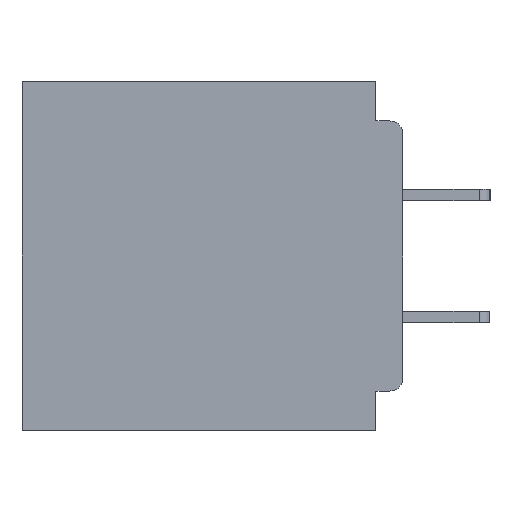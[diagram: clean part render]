
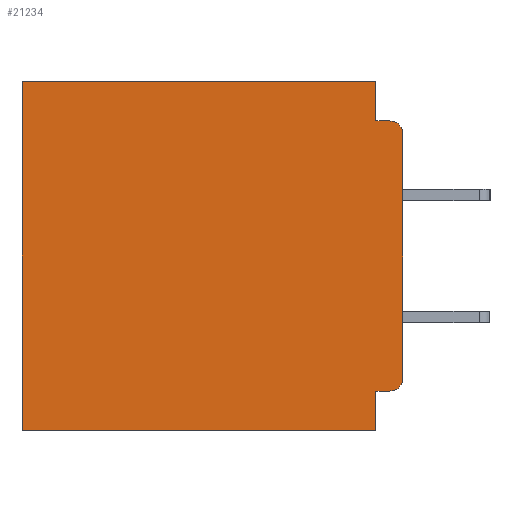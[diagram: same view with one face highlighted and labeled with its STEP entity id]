
A CAD part, left-side view. The second image highlights one B-rep face of the part: STEP entity #21234.
In plain terms, the highlighted planar face has unit normal (-1, 0, 0).
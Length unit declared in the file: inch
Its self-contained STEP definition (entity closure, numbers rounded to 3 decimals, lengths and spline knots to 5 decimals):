
#2300 = CARTESIAN_POINT ( 'NONE',  ( 0.3, 0.437, 0. ) ) ;
#2632 = LINE ( 'NONE', #42427, #29179 ) ;
#2693 = VECTOR ( 'NONE', #25882, 39.37008 ) ;
#2869 = LINE ( 'NONE', #5137, #19590 ) ;
#3194 = VECTOR ( 'NONE', #10880, 39.37008 ) ;
#4747 = CARTESIAN_POINT ( 'NONE',  ( 0.3, 0., -0.34 ) ) ;
#5137 = CARTESIAN_POINT ( 'NONE',  ( 0.3, 0.031, 0. ) ) ;
#5235 = CARTESIAN_POINT ( 'NONE',  ( 0.3, 0.031, -0.355 ) ) ;
#5627 = ORIENTED_EDGE ( 'NONE', *, *, #32504, .T. ) ;
#6073 = AXIS2_PLACEMENT_3D ( 'NONE', #10382, #33582, #13724 ) ;
#6361 = EDGE_CURVE ( 'NONE', #37225, #25148, #37758, .T. ) ;
#6694 = ORIENTED_EDGE ( 'NONE', *, *, #37933, .F. ) ;
#7523 = CARTESIAN_POINT ( 'NONE',  ( 0.3, 0.437, -0.4 ) ) ;
#7629 = EDGE_CURVE ( 'NONE', #35287, #28672, #38664, .T. ) ;
#8501 = DIRECTION ( 'NONE',  ( 0., 0., -1. ) ) ;
#8754 = ORIENTED_EDGE ( 'NONE', *, *, #33433, .T. ) ;
#9682 = VERTEX_POINT ( 'NONE', #33207 ) ;
#10018 = EDGE_CURVE ( 'NONE', #11130, #35287, #2869, .T. ) ;
#10382 = CARTESIAN_POINT ( 'NONE',  ( 0.3, 0., -0.4 ) ) ;
#10880 = DIRECTION ( 'NONE',  ( 0., 0., -1. ) ) ;
#11130 = VERTEX_POINT ( 'NONE', #17285 ) ;
#11133 = CARTESIAN_POINT ( 'NONE',  ( 0.3, 0., -0.4 ) ) ;
#12107 = LINE ( 'NONE', #7523, #3194 ) ;
#12738 = CARTESIAN_POINT ( 'NONE',  ( 0.3, 0., -0.4 ) ) ;
#13204 = VERTEX_POINT ( 'NONE', #5235 ) ;
#13582 = PLANE ( 'NONE',  #6073 ) ;
#13610 = VERTEX_POINT ( 'NONE', #26834 ) ;
#13724 = DIRECTION ( 'NONE',  ( 0., 0., -1. ) ) ;
#14297 = FACE_OUTER_BOUND ( 'NONE', #39934, .T. ) ;
#15374 = VERTEX_POINT ( 'NONE', #38486 ) ;
#17285 = CARTESIAN_POINT ( 'NONE',  ( 0.3, 0.031, 0. ) ) ;
#17609 = DIRECTION ( 'NONE',  ( -1., 0., 0. ) ) ;
#17786 = CARTESIAN_POINT ( 'NONE',  ( 0.3, 0.015, -0.06 ) ) ;
#17788 = LINE ( 'NONE', #22498, #34378 ) ;
#18464 = EDGE_CURVE ( 'NONE', #13610, #25148, #25874, .T. ) ;
#18761 = LINE ( 'NONE', #11133, #26536 ) ;
#19590 = VECTOR ( 'NONE', #8501, 39.37008 ) ;
#19811 = EDGE_CURVE ( 'NONE', #37225, #28672, #27363, .T. ) ;
#20032 = VECTOR ( 'NONE', #39133, 39.37008 ) ;
#20236 = ORIENTED_EDGE ( 'NONE', *, *, #40316, .F. ) ;
#21152 = DIRECTION ( 'NONE',  ( 0., 0., -1. ) ) ;
#21234 = ADVANCED_FACE ( 'NONE', ( #14297 ), #13582, .F. ) ;
#22498 = CARTESIAN_POINT ( 'NONE',  ( 0.3, 0.031, -0.4 ) ) ;
#23610 = AXIS2_PLACEMENT_3D ( 'NONE', #17786, #40914, #21152 ) ;
#25148 = VERTEX_POINT ( 'NONE', #4747 ) ;
#25803 = DIRECTION ( 'NONE',  ( 0., 0., -1. ) ) ;
#25874 = CIRCLE ( 'NONE', #40973, 0.015 ) ;
#25882 = DIRECTION ( 'NONE',  ( 0., 1., 0. ) ) ;
#25914 = ORIENTED_EDGE ( 'NONE', *, *, #28213, .F. ) ;
#26536 = VECTOR ( 'NONE', #31124, 39.37008 ) ;
#26834 = CARTESIAN_POINT ( 'NONE',  ( 0.3, 0.015, -0.355 ) ) ;
#26865 = VECTOR ( 'NONE', #29555, 39.37008 ) ;
#27363 = CIRCLE ( 'NONE', #23610, 0.015 ) ;
#28213 = EDGE_CURVE ( 'NONE', #15374, #9682, #18761, .T. ) ;
#28672 = VERTEX_POINT ( 'NONE', #30220 ) ;
#28886 = ORIENTED_EDGE ( 'NONE', *, *, #6361, .F. ) ;
#29179 = VECTOR ( 'NONE', #35832, 39.37008 ) ;
#29555 = DIRECTION ( 'NONE',  ( 0., 0., -1. ) ) ;
#30220 = CARTESIAN_POINT ( 'NONE',  ( 0.3, 0.015, -0.045 ) ) ;
#31124 = DIRECTION ( 'NONE',  ( 0., 1., 0. ) ) ;
#32504 = EDGE_CURVE ( 'NONE', #11130, #39036, #38049, .T. ) ;
#33207 = CARTESIAN_POINT ( 'NONE',  ( 0.3, 0.437, -0.4 ) ) ;
#33433 = EDGE_CURVE ( 'NONE', #39036, #9682, #12107, .T. ) ;
#33582 = DIRECTION ( 'NONE',  ( 1., 0., 0. ) ) ;
#34378 = VECTOR ( 'NONE', #25803, 39.37008 ) ;
#35287 = VERTEX_POINT ( 'NONE', #38877 ) ;
#35832 = DIRECTION ( 'NONE',  ( 0., 1., 0. ) ) ;
#36218 = ORIENTED_EDGE ( 'NONE', *, *, #10018, .F. ) ;
#37225 = VERTEX_POINT ( 'NONE', #41882 ) ;
#37477 = CARTESIAN_POINT ( 'NONE',  ( 0.3, 0.015, -0.34 ) ) ;
#37758 = LINE ( 'NONE', #12738, #26865 ) ;
#37933 = EDGE_CURVE ( 'NONE', #13610, #13204, #2632, .T. ) ;
#38049 = LINE ( 'NONE', #39033, #2693 ) ;
#38364 = ORIENTED_EDGE ( 'NONE', *, *, #18464, .T. ) ;
#38486 = CARTESIAN_POINT ( 'NONE',  ( 0.3, 0.031, -0.4 ) ) ;
#38664 = LINE ( 'NONE', #42414, #20032 ) ;
#38877 = CARTESIAN_POINT ( 'NONE',  ( 0.3, 0.031, -0.045 ) ) ;
#39033 = CARTESIAN_POINT ( 'NONE',  ( 0.3, 0., 0. ) ) ;
#39036 = VERTEX_POINT ( 'NONE', #2300 ) ;
#39133 = DIRECTION ( 'NONE',  ( 0., -1., 0. ) ) ;
#39934 = EDGE_LOOP ( 'NONE', ( #28886, #41301, #41851, #36218, #5627, #8754, #25914, #20236, #6694, #38364 ) ) ;
#40316 = EDGE_CURVE ( 'NONE', #13204, #15374, #17788, .T. ) ;
#40735 = DIRECTION ( 'NONE',  ( 0., 0., -1. ) ) ;
#40914 = DIRECTION ( 'NONE',  ( -1., 0., 0. ) ) ;
#40973 = AXIS2_PLACEMENT_3D ( 'NONE', #37477, #17609, #40735 ) ;
#41301 = ORIENTED_EDGE ( 'NONE', *, *, #19811, .T. ) ;
#41851 = ORIENTED_EDGE ( 'NONE', *, *, #7629, .F. ) ;
#41882 = CARTESIAN_POINT ( 'NONE',  ( 0.3, 0., -0.06 ) ) ;
#42414 = CARTESIAN_POINT ( 'NONE',  ( 0.3, 0., -0.045 ) ) ;
#42427 = CARTESIAN_POINT ( 'NONE',  ( 0.3, 0., -0.355 ) ) ;
